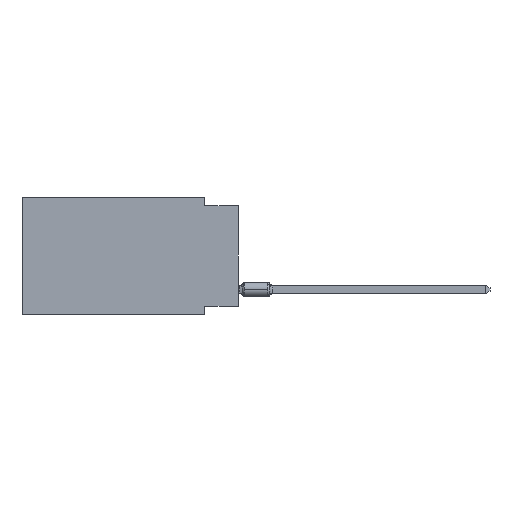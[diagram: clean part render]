
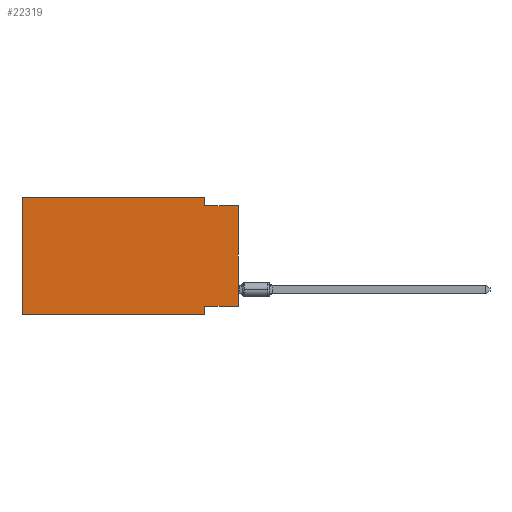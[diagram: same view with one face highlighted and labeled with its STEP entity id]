
A CAD part, left-side view. The second image highlights one B-rep face of the part: STEP entity #22319.
In plain terms, the highlighted planar face has unit normal (-1, 0, 0).
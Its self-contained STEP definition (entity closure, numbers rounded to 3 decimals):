
#552 = CARTESIAN_POINT ( 'NONE',  ( 0., 16.383, 0. ) ) ;
#679 = CARTESIAN_POINT ( 'NONE',  ( 0., 0., 0. ) ) ;
#745 = ORIENTED_EDGE ( 'NONE', *, *, #4967, .F. ) ;
#1742 = ORIENTED_EDGE ( 'NONE', *, *, #20322, .T. ) ;
#1962 = VERTEX_POINT ( 'NONE', #15761 ) ;
#1998 = CARTESIAN_POINT ( 'NONE',  ( 0., 2.54, 0. ) ) ;
#2160 = CARTESIAN_POINT ( 'NONE',  ( 0., 16.383, 0. ) ) ;
#2309 = VECTOR ( 'NONE', #12159, 1000. ) ;
#2887 = CARTESIAN_POINT ( 'NONE',  ( 0., 0., -0.635 ) ) ;
#3197 = EDGE_CURVE ( 'NONE', #12890, #20580, #4238, .T. ) ;
#3469 = DIRECTION ( 'NONE',  ( 0., 0., -1. ) ) ;
#3558 = ORIENTED_EDGE ( 'NONE', *, *, #17709, .T. ) ;
#4022 = EDGE_CURVE ( 'NONE', #4496, #17626, #13334, .T. ) ;
#4238 = LINE ( 'NONE', #7810, #21649 ) ;
#4496 = VERTEX_POINT ( 'NONE', #13513 ) ;
#4551 = EDGE_CURVE ( 'NONE', #16155, #12890, #4664, .T. ) ;
#4664 = LINE ( 'NONE', #6864, #13862 ) ;
#4967 = EDGE_CURVE ( 'NONE', #1962, #16792, #6241, .T. ) ;
#5323 = DIRECTION ( 'NONE',  ( 0., 0., -1. ) ) ;
#5973 = CARTESIAN_POINT ( 'NONE',  ( 0., 2.54, -8.89 ) ) ;
#6241 = LINE ( 'NONE', #2887, #15067 ) ;
#6279 = CARTESIAN_POINT ( 'NONE',  ( 0., 16.383, -8.89 ) ) ;
#6607 = CARTESIAN_POINT ( 'NONE',  ( 0., 2.54, 0. ) ) ;
#6685 = LINE ( 'NONE', #12210, #14337 ) ;
#6804 = DIRECTION ( 'NONE',  ( 0., -1., 0. ) ) ;
#6864 = CARTESIAN_POINT ( 'NONE',  ( 0., 0., -8.255 ) ) ;
#7419 = FACE_OUTER_BOUND ( 'NONE', #18488, .T. ) ;
#7810 = CARTESIAN_POINT ( 'NONE',  ( 0., 2.54, -8.89 ) ) ;
#8685 = EDGE_CURVE ( 'NONE', #17626, #13242, #6685, .T. ) ;
#8893 = CARTESIAN_POINT ( 'NONE',  ( 0., 16.383, 0. ) ) ;
#9532 = DIRECTION ( 'NONE',  ( 0., 0., 1. ) ) ;
#9792 = DIRECTION ( 'NONE',  ( 0., 0., 1. ) ) ;
#9946 = VECTOR ( 'NONE', #9532, 1000. ) ;
#10166 = DIRECTION ( 'NONE',  ( 0., -1., 0. ) ) ;
#10930 = EDGE_CURVE ( 'NONE', #13242, #1962, #20285, .T. ) ;
#11633 = ORIENTED_EDGE ( 'NONE', *, *, #4551, .F. ) ;
#12159 = DIRECTION ( 'NONE',  ( 0., -1., 0. ) ) ;
#12210 = CARTESIAN_POINT ( 'NONE',  ( 0., 16.383, 0. ) ) ;
#12262 = DIRECTION ( 'NONE',  ( 0., 1., 0. ) ) ;
#12890 = VERTEX_POINT ( 'NONE', #22315 ) ;
#13242 = VERTEX_POINT ( 'NONE', #6607 ) ;
#13334 = LINE ( 'NONE', #2160, #9946 ) ;
#13513 = CARTESIAN_POINT ( 'NONE',  ( 0., 16.383, -8.89 ) ) ;
#13577 = AXIS2_PLACEMENT_3D ( 'NONE', #8893, #23731, #5323 ) ;
#13862 = VECTOR ( 'NONE', #12262, 1000. ) ;
#14337 = VECTOR ( 'NONE', #6804, 1000. ) ;
#14371 = VECTOR ( 'NONE', #9792, 1000. ) ;
#14643 = PLANE ( 'NONE',  #13577 ) ;
#15067 = VECTOR ( 'NONE', #10166, 1000. ) ;
#15761 = CARTESIAN_POINT ( 'NONE',  ( 0., 2.54, -0.635 ) ) ;
#16155 = VERTEX_POINT ( 'NONE', #19315 ) ;
#16792 = VERTEX_POINT ( 'NONE', #22217 ) ;
#17626 = VERTEX_POINT ( 'NONE', #552 ) ;
#17709 = EDGE_CURVE ( 'NONE', #16155, #16792, #19225, .T. ) ;
#17907 = LINE ( 'NONE', #6279, #2309 ) ;
#18488 = EDGE_LOOP ( 'NONE', ( #3558, #745, #22859, #23303, #22698, #1742, #21447, #11633 ) ) ;
#19225 = LINE ( 'NONE', #679, #14371 ) ;
#19315 = CARTESIAN_POINT ( 'NONE',  ( 0., 0., -8.255 ) ) ;
#20285 = LINE ( 'NONE', #1998, #22302 ) ;
#20322 = EDGE_CURVE ( 'NONE', #4496, #20580, #17907, .T. ) ;
#20580 = VERTEX_POINT ( 'NONE', #5973 ) ;
#21447 = ORIENTED_EDGE ( 'NONE', *, *, #3197, .F. ) ;
#21649 = VECTOR ( 'NONE', #22770, 1000. ) ;
#22217 = CARTESIAN_POINT ( 'NONE',  ( 0., 0., -0.635 ) ) ;
#22302 = VECTOR ( 'NONE', #3469, 1000. ) ;
#22315 = CARTESIAN_POINT ( 'NONE',  ( 0., 2.54, -8.255 ) ) ;
#22319 = ADVANCED_FACE ( 'NONE', ( #7419 ), #14643, .F. ) ;
#22698 = ORIENTED_EDGE ( 'NONE', *, *, #4022, .F. ) ;
#22770 = DIRECTION ( 'NONE',  ( 0., 0., -1. ) ) ;
#22859 = ORIENTED_EDGE ( 'NONE', *, *, #10930, .F. ) ;
#23303 = ORIENTED_EDGE ( 'NONE', *, *, #8685, .F. ) ;
#23731 = DIRECTION ( 'NONE',  ( 1., 0., 0. ) ) ;
